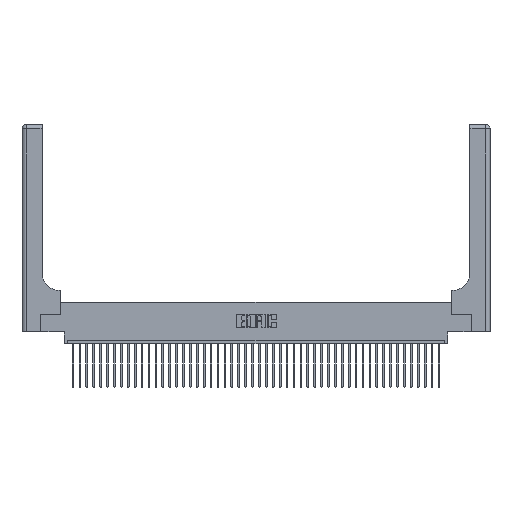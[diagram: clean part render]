
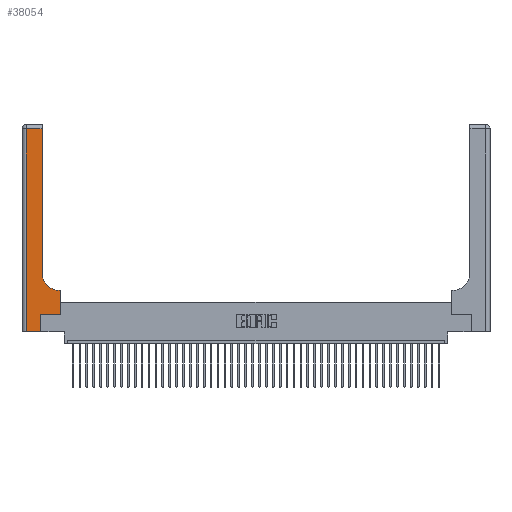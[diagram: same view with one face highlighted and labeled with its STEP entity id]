
A CAD part, top view. The second image highlights one B-rep face of the part: STEP entity #38054.
In plain terms, the highlighted planar face has unit normal (0, 0, 1).
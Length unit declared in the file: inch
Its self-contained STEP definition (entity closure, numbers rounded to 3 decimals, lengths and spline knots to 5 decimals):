
#12 = CIRCLE ( 'NONE', #34584, 0.25 ) ;
#110 = CARTESIAN_POINT ( 'NONE',  ( 0.2915, 0.85, 0.37 ) ) ;
#875 = VERTEX_POINT ( 'NONE', #10387 ) ;
#2198 = CARTESIAN_POINT ( 'NONE',  ( 0.06, 3., 0.37 ) ) ;
#2433 = DIRECTION ( 'NONE',  ( -1., 0., 0. ) ) ;
#2879 = VERTEX_POINT ( 'NONE', #9890 ) ;
#4140 = VERTEX_POINT ( 'NONE', #39319 ) ;
#4424 = ORIENTED_EDGE ( 'NONE', *, *, #24193, .T. ) ;
#5722 = DIRECTION ( 'NONE',  ( 0., 0., -1. ) ) ;
#6802 = EDGE_LOOP ( 'NONE', ( #17479, #4424, #18391, #28629, #37854, #37124, #8384, #24135, #36146 ) ) ;
#8384 = ORIENTED_EDGE ( 'NONE', *, *, #39796, .T. ) ;
#9044 = LINE ( 'NONE', #2198, #28825 ) ;
#9890 = CARTESIAN_POINT ( 'NONE',  ( 0.5585, 0.6, 0.37 ) ) ;
#9924 = CARTESIAN_POINT ( 'NONE',  ( 0.269, 0., 0.37 ) ) ;
#10284 = VECTOR ( 'NONE', #17540, 39.37008 ) ;
#10321 = AXIS2_PLACEMENT_3D ( 'NONE', #25928, #26081, #20093 ) ;
#10387 = CARTESIAN_POINT ( 'NONE',  ( 0.2915, 2.94, 0.37 ) ) ;
#11545 = LINE ( 'NONE', #9924, #43684 ) ;
#12456 = CARTESIAN_POINT ( 'NONE',  ( 0.5415, 0.85, 0.37 ) ) ;
#14726 = VECTOR ( 'NONE', #2433, 39.37008 ) ;
#15852 = CARTESIAN_POINT ( 'NONE',  ( 0.06, 2.94, 0.37 ) ) ;
#16638 = PLANE ( 'NONE',  #10321 ) ;
#17317 = CARTESIAN_POINT ( 'NONE',  ( 0., 0., 0.37 ) ) ;
#17479 = ORIENTED_EDGE ( 'NONE', *, *, #37684, .T. ) ;
#17540 = DIRECTION ( 'NONE',  ( -1., 0., 0. ) ) ;
#17763 = LINE ( 'NONE', #17317, #21514 ) ;
#18238 = EDGE_CURVE ( 'NONE', #23746, #36886, #11545, .T. ) ;
#18391 = ORIENTED_EDGE ( 'NONE', *, *, #43935, .T. ) ;
#19331 = DIRECTION ( 'NONE',  ( 1., 0., 0. ) ) ;
#19713 = EDGE_CURVE ( 'NONE', #36886, #35413, #39253, .T. ) ;
#20093 = DIRECTION ( 'NONE',  ( -1., 0., 0. ) ) ;
#20797 = LINE ( 'NONE', #41463, #24535 ) ;
#21016 = CARTESIAN_POINT ( 'NONE',  ( 0.5585, 0.25, 0.37 ) ) ;
#21278 = EDGE_CURVE ( 'NONE', #4140, #24882, #12, .T. ) ;
#21514 = VECTOR ( 'NONE', #41588, 39.37008 ) ;
#22609 = FACE_OUTER_BOUND ( 'NONE', #6802, .T. ) ;
#22641 = DIRECTION ( 'NONE',  ( 0., 1., 0. ) ) ;
#22875 = EDGE_CURVE ( 'NONE', #2879, #4140, #28495, .T. ) ;
#23620 = VERTEX_POINT ( 'NONE', #15852 ) ;
#23746 = VERTEX_POINT ( 'NONE', #40692 ) ;
#24135 = ORIENTED_EDGE ( 'NONE', *, *, #22875, .T. ) ;
#24193 = EDGE_CURVE ( 'NONE', #875, #23620, #33697, .T. ) ;
#24535 = VECTOR ( 'NONE', #24671, 39.37008 ) ;
#24671 = DIRECTION ( 'NONE',  ( 0., 1., 0. ) ) ;
#24882 = VERTEX_POINT ( 'NONE', #110 ) ;
#25030 = CARTESIAN_POINT ( 'NONE',  ( 0.2915, 0.6, 0.37 ) ) ;
#25928 = CARTESIAN_POINT ( 'NONE',  ( 0., 3., 0.37 ) ) ;
#26081 = DIRECTION ( 'NONE',  ( 0., 0., -1. ) ) ;
#26232 = DIRECTION ( 'NONE',  ( 0., -1., 0. ) ) ;
#26370 = VECTOR ( 'NONE', #37381, 39.37008 ) ;
#27431 = DIRECTION ( 'NONE',  ( 0., 1., 0. ) ) ;
#28495 = LINE ( 'NONE', #25030, #10284 ) ;
#28629 = ORIENTED_EDGE ( 'NONE', *, *, #29946, .T. ) ;
#28825 = VECTOR ( 'NONE', #26232, 39.37008 ) ;
#29905 = CARTESIAN_POINT ( 'NONE',  ( 0., 2.94, 0.37 ) ) ;
#29946 = EDGE_CURVE ( 'NONE', #31637, #23746, #17763, .T. ) ;
#31637 = VERTEX_POINT ( 'NONE', #43550 ) ;
#33697 = LINE ( 'NONE', #29905, #14726 ) ;
#34492 = CARTESIAN_POINT ( 'NONE',  ( 0.269, 0.25, 0.37 ) ) ;
#34584 = AXIS2_PLACEMENT_3D ( 'NONE', #12456, #5722, #19331 ) ;
#35413 = VERTEX_POINT ( 'NONE', #21016 ) ;
#36146 = ORIENTED_EDGE ( 'NONE', *, *, #21278, .T. ) ;
#36886 = VERTEX_POINT ( 'NONE', #43412 ) ;
#37124 = ORIENTED_EDGE ( 'NONE', *, *, #19713, .T. ) ;
#37366 = CARTESIAN_POINT ( 'NONE',  ( 0.2915, 3., 0.37 ) ) ;
#37381 = DIRECTION ( 'NONE',  ( 1., 0., 0. ) ) ;
#37684 = EDGE_CURVE ( 'NONE', #24882, #875, #41382, .T. ) ;
#37854 = ORIENTED_EDGE ( 'NONE', *, *, #18238, .T. ) ;
#38054 = ADVANCED_FACE ( 'NONE', ( #22609 ), #16638, .F. ) ;
#39253 = LINE ( 'NONE', #34492, #26370 ) ;
#39319 = CARTESIAN_POINT ( 'NONE',  ( 0.5415, 0.6, 0.37 ) ) ;
#39796 = EDGE_CURVE ( 'NONE', #35413, #2879, #20797, .T. ) ;
#40692 = CARTESIAN_POINT ( 'NONE',  ( 0.269, 0., 0.37 ) ) ;
#41382 = LINE ( 'NONE', #37366, #43024 ) ;
#41463 = CARTESIAN_POINT ( 'NONE',  ( 0.5585, 0.25, 0.37 ) ) ;
#41588 = DIRECTION ( 'NONE',  ( 1., 0., 0. ) ) ;
#43024 = VECTOR ( 'NONE', #27431, 39.37008 ) ;
#43412 = CARTESIAN_POINT ( 'NONE',  ( 0.269, 0.25, 0.37 ) ) ;
#43550 = CARTESIAN_POINT ( 'NONE',  ( 0.06, 0., 0.37 ) ) ;
#43684 = VECTOR ( 'NONE', #22641, 39.37008 ) ;
#43935 = EDGE_CURVE ( 'NONE', #23620, #31637, #9044, .T. ) ;
